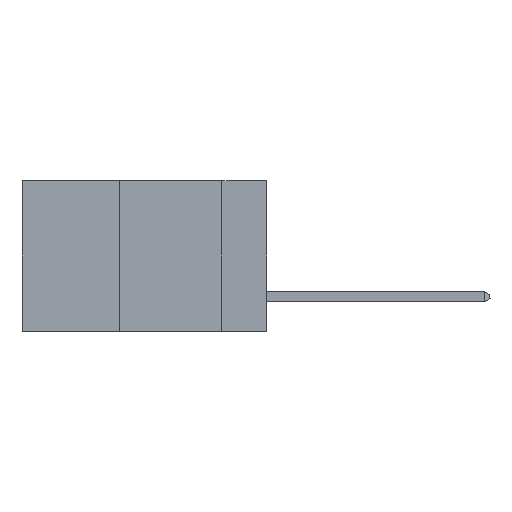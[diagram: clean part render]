
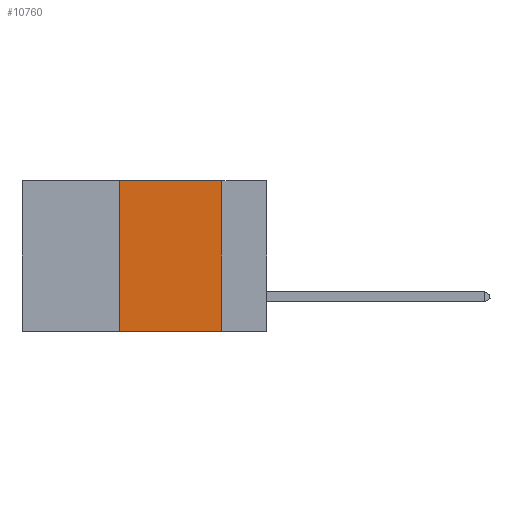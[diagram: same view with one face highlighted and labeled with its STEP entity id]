
A CAD part, left-side view. The second image highlights one B-rep face of the part: STEP entity #10760.
In plain terms, the highlighted planar face has unit normal (-1, 0, 0).
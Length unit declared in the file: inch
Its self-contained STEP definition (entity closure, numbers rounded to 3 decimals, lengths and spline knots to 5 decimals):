
#130 = VECTOR ( 'NONE', #6501, 39.37008 ) ;
#393 = ORIENTED_EDGE ( 'NONE', *, *, #12920, .F. ) ;
#809 = LINE ( 'NONE', #7498, #130 ) ;
#1094 = PLANE ( 'NONE',  #5648 ) ;
#1758 = EDGE_LOOP ( 'NONE', ( #393, #10370, #9054, #6292 ) ) ;
#3093 = DIRECTION ( 'NONE',  ( 0., -1., 0. ) ) ;
#3744 = CARTESIAN_POINT ( 'NONE',  ( 0., 0.11, 0. ) ) ;
#4121 = LINE ( 'NONE', #3744, #9625 ) ;
#4258 = CARTESIAN_POINT ( 'NONE',  ( 0., 0.6, 0. ) ) ;
#4872 = DIRECTION ( 'NONE',  ( 0., -1., 0. ) ) ;
#4975 = VERTEX_POINT ( 'NONE', #5742 ) ;
#5543 = EDGE_CURVE ( 'NONE', #8074, #4975, #10857, .T. ) ;
#5633 = VECTOR ( 'NONE', #3093, 39.37008 ) ;
#5648 = AXIS2_PLACEMENT_3D ( 'NONE', #4258, #6417, #9590 ) ;
#5710 = CARTESIAN_POINT ( 'NONE',  ( 0., 0.6, 0. ) ) ;
#5742 = CARTESIAN_POINT ( 'NONE',  ( 0., 0.11, -0.37 ) ) ;
#5869 = VERTEX_POINT ( 'NONE', #12862 ) ;
#6292 = ORIENTED_EDGE ( 'NONE', *, *, #5543, .T. ) ;
#6417 = DIRECTION ( 'NONE',  ( 1., 0., 0. ) ) ;
#6501 = DIRECTION ( 'NONE',  ( 0., 0., 1. ) ) ;
#6568 = EDGE_CURVE ( 'NONE', #5869, #8554, #8502, .T. ) ;
#6650 = VECTOR ( 'NONE', #4872, 39.37008 ) ;
#6708 = FACE_OUTER_BOUND ( 'NONE', #1758, .T. ) ;
#7498 = CARTESIAN_POINT ( 'NONE',  ( 0., 0.36, 0. ) ) ;
#8074 = VERTEX_POINT ( 'NONE', #11571 ) ;
#8260 = EDGE_CURVE ( 'NONE', #8074, #5869, #809, .T. ) ;
#8502 = LINE ( 'NONE', #5710, #5633 ) ;
#8554 = VERTEX_POINT ( 'NONE', #11474 ) ;
#9054 = ORIENTED_EDGE ( 'NONE', *, *, #8260, .F. ) ;
#9590 = DIRECTION ( 'NONE',  ( 0., 0., -1. ) ) ;
#9625 = VECTOR ( 'NONE', #13511, 39.37008 ) ;
#10370 = ORIENTED_EDGE ( 'NONE', *, *, #6568, .F. ) ;
#10760 = ADVANCED_FACE ( 'NONE', ( #6708 ), #1094, .F. ) ;
#10857 = LINE ( 'NONE', #11308, #6650 ) ;
#11308 = CARTESIAN_POINT ( 'NONE',  ( 0., 0.6, -0.37 ) ) ;
#11474 = CARTESIAN_POINT ( 'NONE',  ( 0., 0.11, 0. ) ) ;
#11571 = CARTESIAN_POINT ( 'NONE',  ( 0., 0.36, -0.37 ) ) ;
#12862 = CARTESIAN_POINT ( 'NONE',  ( 0., 0.36, 0. ) ) ;
#12920 = EDGE_CURVE ( 'NONE', #8554, #4975, #4121, .T. ) ;
#13511 = DIRECTION ( 'NONE',  ( 0., 0., -1. ) ) ;
